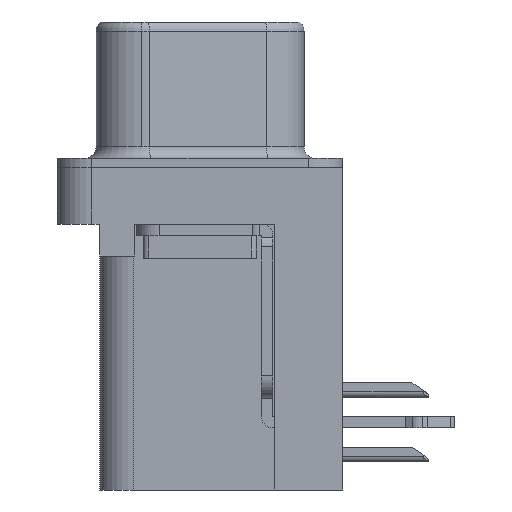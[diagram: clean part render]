
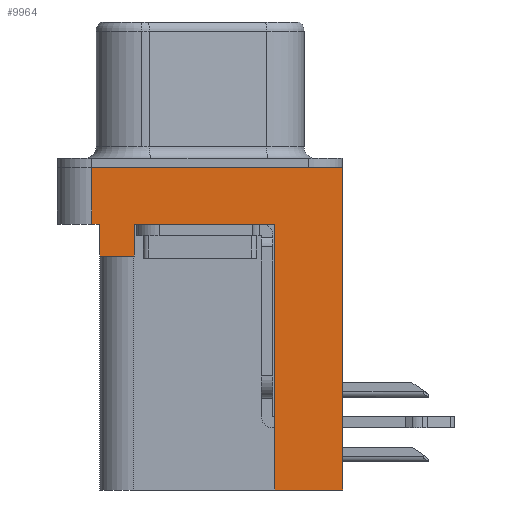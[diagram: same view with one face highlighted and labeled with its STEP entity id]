
A CAD part, left-side view. The second image highlights one B-rep face of the part: STEP entity #9964.
In plain terms, the highlighted planar face has unit normal (-1, 0, 0).
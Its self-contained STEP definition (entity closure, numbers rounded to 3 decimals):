
#120 = EDGE_CURVE ( 'NONE', #2723, #10780, #6781, .T. ) ;
#198 = DIRECTION ( 'NONE',  ( 0., 0., 1. ) ) ;
#231 = ORIENTED_EDGE ( 'NONE', *, *, #3459, .T. ) ;
#499 = CARTESIAN_POINT ( 'NONE',  ( -2.935, -3.295, -14.2 ) ) ;
#802 = ORIENTED_EDGE ( 'NONE', *, *, #16605, .T. ) ;
#1219 = CARTESIAN_POINT ( 'NONE',  ( -2.935, 4.775, 0. ) ) ;
#1335 = VECTOR ( 'NONE', #15937, 1000. ) ;
#1377 = CARTESIAN_POINT ( 'NONE',  ( -2.935, 2.895, -2.5 ) ) ;
#2322 = DIRECTION ( 'NONE',  ( 0., -1., 0. ) ) ;
#2496 = CARTESIAN_POINT ( 'NONE',  ( -2.935, -6.275, -2.5 ) ) ;
#2695 = ORIENTED_EDGE ( 'NONE', *, *, #3743, .T. ) ;
#2723 = VERTEX_POINT ( 'NONE', #14109 ) ;
#2726 = CARTESIAN_POINT ( 'NONE',  ( -2.935, -6.275, -2.5 ) ) ;
#2820 = FACE_OUTER_BOUND ( 'NONE', #3853, .T. ) ;
#2855 = CARTESIAN_POINT ( 'NONE',  ( -2.935, -6.275, -2.5 ) ) ;
#2892 = LINE ( 'NONE', #6910, #9624 ) ;
#3431 = CARTESIAN_POINT ( 'NONE',  ( -2.935, 4.775, -2.5 ) ) ;
#3459 = EDGE_CURVE ( 'NONE', #10780, #12005, #13166, .T. ) ;
#3611 = CARTESIAN_POINT ( 'NONE',  ( -2.935, -6.275, 0. ) ) ;
#3743 = EDGE_CURVE ( 'NONE', #13077, #4744, #4084, .T. ) ;
#3750 = CARTESIAN_POINT ( 'NONE',  ( -2.935, 4.425, -2.5 ) ) ;
#3774 = VECTOR ( 'NONE', #9239, 1000. ) ;
#3823 = ORIENTED_EDGE ( 'NONE', *, *, #9159, .F. ) ;
#3853 = EDGE_LOOP ( 'NONE', ( #10748, #14322, #2695, #4317, #16908, #11357, #231, #3823, #3981, #802 ) ) ;
#3865 = VECTOR ( 'NONE', #7584, 1000. ) ;
#3981 = ORIENTED_EDGE ( 'NONE', *, *, #10361, .F. ) ;
#4084 = LINE ( 'NONE', #2855, #13389 ) ;
#4094 = LINE ( 'NONE', #11865, #3774 ) ;
#4317 = ORIENTED_EDGE ( 'NONE', *, *, #16173, .F. ) ;
#4405 = PLANE ( 'NONE',  #16602 ) ;
#4530 = DIRECTION ( 'NONE',  ( 0., 0., 1. ) ) ;
#4656 = VERTEX_POINT ( 'NONE', #14969 ) ;
#4744 = VERTEX_POINT ( 'NONE', #3750 ) ;
#4905 = VERTEX_POINT ( 'NONE', #11986 ) ;
#5100 = LINE ( 'NONE', #3611, #11268 ) ;
#5955 = VECTOR ( 'NONE', #4530, 1000. ) ;
#6118 = VECTOR ( 'NONE', #2322, 1000. ) ;
#6781 = LINE ( 'NONE', #8082, #7858 ) ;
#6910 = CARTESIAN_POINT ( 'NONE',  ( -2.935, -3.295, -14.2 ) ) ;
#7169 = VERTEX_POINT ( 'NONE', #1219 ) ;
#7584 = DIRECTION ( 'NONE',  ( 0., 0., 1. ) ) ;
#7858 = VECTOR ( 'NONE', #15005, 1000. ) ;
#7999 = DIRECTION ( 'NONE',  ( 0., -1., 0. ) ) ;
#8082 = CARTESIAN_POINT ( 'NONE',  ( -2.935, 2.895, -3.9 ) ) ;
#8529 = LINE ( 'NONE', #499, #5955 ) ;
#9159 = EDGE_CURVE ( 'NONE', #4656, #12005, #8529, .T. ) ;
#9239 = DIRECTION ( 'NONE',  ( 0., 1., 0. ) ) ;
#9240 = CARTESIAN_POINT ( 'NONE',  ( -2.935, -3.295, -2.5 ) ) ;
#9241 = VERTEX_POINT ( 'NONE', #12812 ) ;
#9624 = VECTOR ( 'NONE', #16277, 1000. ) ;
#9632 = EDGE_CURVE ( 'NONE', #7169, #4905, #5100, .T. ) ;
#9964 = ADVANCED_FACE ( 'NONE', ( #2820 ), #4405, .T. ) ;
#10226 = LINE ( 'NONE', #16953, #3865 ) ;
#10361 = EDGE_CURVE ( 'NONE', #11503, #4656, #2892, .T. ) ;
#10522 = CARTESIAN_POINT ( 'NONE',  ( -2.935, 4.775, -2.5 ) ) ;
#10748 = ORIENTED_EDGE ( 'NONE', *, *, #9632, .F. ) ;
#10780 = VERTEX_POINT ( 'NONE', #1377 ) ;
#10882 = EDGE_CURVE ( 'NONE', #2723, #9241, #4094, .T. ) ;
#11268 = VECTOR ( 'NONE', #16734, 1000. ) ;
#11357 = ORIENTED_EDGE ( 'NONE', *, *, #120, .T. ) ;
#11503 = VERTEX_POINT ( 'NONE', #13771 ) ;
#11865 = CARTESIAN_POINT ( 'NONE',  ( -2.935, 4.425, -3.9 ) ) ;
#11986 = CARTESIAN_POINT ( 'NONE',  ( -2.935, -6.275, 0. ) ) ;
#12005 = VERTEX_POINT ( 'NONE', #9240 ) ;
#12091 = DIRECTION ( 'NONE',  ( -1., 0., 0. ) ) ;
#12812 = CARTESIAN_POINT ( 'NONE',  ( -2.935, 4.425, -3.9 ) ) ;
#12872 = CARTESIAN_POINT ( 'NONE',  ( -2.935, 4.425, -3.9 ) ) ;
#13077 = VERTEX_POINT ( 'NONE', #10522 ) ;
#13166 = LINE ( 'NONE', #2496, #6118 ) ;
#13389 = VECTOR ( 'NONE', #7999, 1000. ) ;
#13771 = CARTESIAN_POINT ( 'NONE',  ( -2.935, -6.275, -14.2 ) ) ;
#14109 = CARTESIAN_POINT ( 'NONE',  ( -2.935, 2.895, -3.9 ) ) ;
#14322 = ORIENTED_EDGE ( 'NONE', *, *, #16054, .F. ) ;
#14969 = CARTESIAN_POINT ( 'NONE',  ( -2.935, -3.295, -14.2 ) ) ;
#15005 = DIRECTION ( 'NONE',  ( 0., 0., 1. ) ) ;
#15669 = LINE ( 'NONE', #12872, #1335 ) ;
#15937 = DIRECTION ( 'NONE',  ( 0., 0., 1. ) ) ;
#16054 = EDGE_CURVE ( 'NONE', #13077, #7169, #16650, .T. ) ;
#16173 = EDGE_CURVE ( 'NONE', #9241, #4744, #15669, .T. ) ;
#16277 = DIRECTION ( 'NONE',  ( 0., 1., 0. ) ) ;
#16478 = DIRECTION ( 'NONE',  ( 0., 0., 1. ) ) ;
#16602 = AXIS2_PLACEMENT_3D ( 'NONE', #2726, #12091, #198 ) ;
#16605 = EDGE_CURVE ( 'NONE', #11503, #4905, #10226, .T. ) ;
#16650 = LINE ( 'NONE', #3431, #16700 ) ;
#16700 = VECTOR ( 'NONE', #16478, 1000. ) ;
#16734 = DIRECTION ( 'NONE',  ( 0., -1., 0. ) ) ;
#16908 = ORIENTED_EDGE ( 'NONE', *, *, #10882, .F. ) ;
#16953 = CARTESIAN_POINT ( 'NONE',  ( -2.935, -6.275, -2.5 ) ) ;
